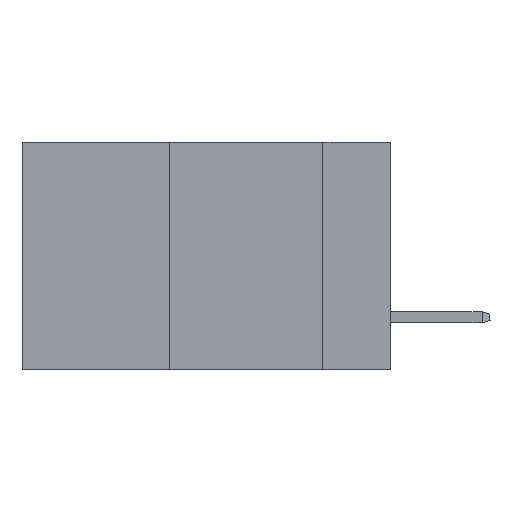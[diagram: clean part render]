
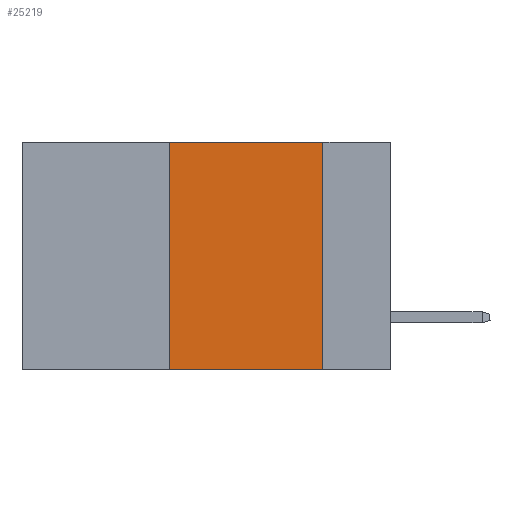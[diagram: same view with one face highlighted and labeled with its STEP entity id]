
A CAD part, left-side view. The second image highlights one B-rep face of the part: STEP entity #25219.
In plain terms, the highlighted planar face has unit normal (-1, 0, 0).
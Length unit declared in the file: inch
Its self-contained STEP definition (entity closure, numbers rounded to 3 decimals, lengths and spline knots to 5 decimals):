
#582 = FACE_OUTER_BOUND ( 'NONE', #42343, .T. ) ;
#936 = VECTOR ( 'NONE', #21588, 39.37008 ) ;
#3787 = EDGE_CURVE ( 'NONE', #29418, #39351, #39235, .T. ) ;
#4880 = CARTESIAN_POINT ( 'NONE',  ( 0., 0.6, 0. ) ) ;
#5631 = VECTOR ( 'NONE', #13753, 39.37008 ) ;
#6498 = ORIENTED_EDGE ( 'NONE', *, *, #26865, .F. ) ;
#6935 = CARTESIAN_POINT ( 'NONE',  ( 0., 0.36, 0. ) ) ;
#9187 = DIRECTION ( 'NONE',  ( 0., -1., 0. ) ) ;
#11845 = EDGE_CURVE ( 'NONE', #29418, #21660, #33747, .T. ) ;
#13346 = CARTESIAN_POINT ( 'NONE',  ( 0., 0.11, -0.37 ) ) ;
#13753 = DIRECTION ( 'NONE',  ( 0., -1., 0. ) ) ;
#16024 = DIRECTION ( 'NONE',  ( 1., 0., 0. ) ) ;
#17898 = VECTOR ( 'NONE', #9187, 39.37008 ) ;
#21454 = LINE ( 'NONE', #38683, #32162 ) ;
#21588 = DIRECTION ( 'NONE',  ( 0., 0., 1. ) ) ;
#21629 = CARTESIAN_POINT ( 'NONE',  ( 0., 0.36, -0.37 ) ) ;
#21660 = VERTEX_POINT ( 'NONE', #13346 ) ;
#25219 = ADVANCED_FACE ( 'NONE', ( #582 ), #26457, .F. ) ;
#25627 = AXIS2_PLACEMENT_3D ( 'NONE', #4880, #16024, #44872 ) ;
#26457 = PLANE ( 'NONE',  #25627 ) ;
#26865 = EDGE_CURVE ( 'NONE', #39351, #34598, #36479, .T. ) ;
#29418 = VERTEX_POINT ( 'NONE', #21629 ) ;
#30588 = CARTESIAN_POINT ( 'NONE',  ( 0., 0.6, 0. ) ) ;
#32162 = VECTOR ( 'NONE', #45964, 39.37008 ) ;
#33747 = LINE ( 'NONE', #46081, #5631 ) ;
#34598 = VERTEX_POINT ( 'NONE', #46623 ) ;
#35234 = ORIENTED_EDGE ( 'NONE', *, *, #3787, .F. ) ;
#36479 = LINE ( 'NONE', #30588, #17898 ) ;
#37635 = ORIENTED_EDGE ( 'NONE', *, *, #11845, .T. ) ;
#38683 = CARTESIAN_POINT ( 'NONE',  ( 0., 0.11, 0. ) ) ;
#39235 = LINE ( 'NONE', #6935, #936 ) ;
#39351 = VERTEX_POINT ( 'NONE', #42409 ) ;
#40157 = EDGE_CURVE ( 'NONE', #34598, #21660, #21454, .T. ) ;
#41520 = ORIENTED_EDGE ( 'NONE', *, *, #40157, .F. ) ;
#42343 = EDGE_LOOP ( 'NONE', ( #41520, #6498, #35234, #37635 ) ) ;
#42409 = CARTESIAN_POINT ( 'NONE',  ( 0., 0.36, 0. ) ) ;
#44872 = DIRECTION ( 'NONE',  ( 0., 0., -1. ) ) ;
#45964 = DIRECTION ( 'NONE',  ( 0., 0., -1. ) ) ;
#46081 = CARTESIAN_POINT ( 'NONE',  ( 0., 0.6, -0.37 ) ) ;
#46623 = CARTESIAN_POINT ( 'NONE',  ( 0., 0.11, 0. ) ) ;
